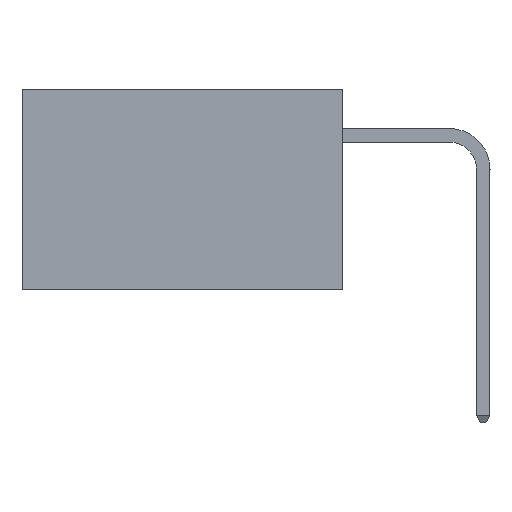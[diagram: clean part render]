
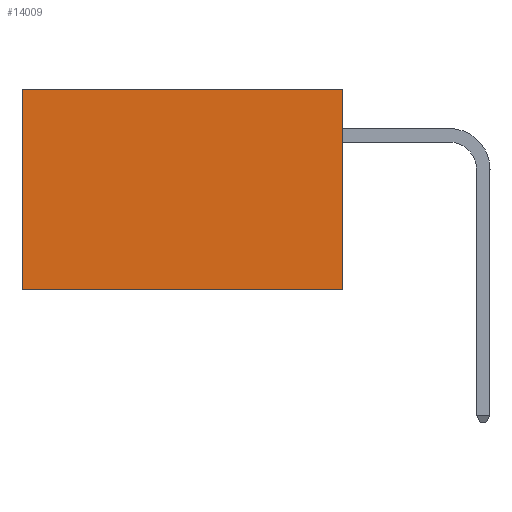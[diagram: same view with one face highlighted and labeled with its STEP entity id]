
A CAD part, left-side view. The second image highlights one B-rep face of the part: STEP entity #14009.
In plain terms, the highlighted planar face has unit normal (-1, 0, 0).
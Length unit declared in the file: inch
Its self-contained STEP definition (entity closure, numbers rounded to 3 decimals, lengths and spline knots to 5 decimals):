
#9 = EDGE_CURVE ( 'NONE', #1036, #16389, #4591, .T. ) ;
#701 = CARTESIAN_POINT ( 'NONE',  ( 0.277, 0., -0.37 ) ) ;
#793 = LINE ( 'NONE', #799, #8828 ) ;
#799 = CARTESIAN_POINT ( 'NONE',  ( 0.277, 0., -0.37 ) ) ;
#1036 = VERTEX_POINT ( 'NONE', #1384 ) ;
#1041 = ORIENTED_EDGE ( 'NONE', *, *, #9, .T. ) ;
#1384 = CARTESIAN_POINT ( 'NONE',  ( 0.277, 0., 0. ) ) ;
#2381 = DIRECTION ( 'NONE',  ( 0., 0., -1. ) ) ;
#2411 = DIRECTION ( 'NONE',  ( 0., 0., -1. ) ) ;
#2448 = DIRECTION ( 'NONE',  ( 0., 1., 0. ) ) ;
#4387 = CARTESIAN_POINT ( 'NONE',  ( 0.277, 0.59, -0.37 ) ) ;
#4591 = LINE ( 'NONE', #5371, #12513 ) ;
#4820 = CARTESIAN_POINT ( 'NONE',  ( 0.277, 0.59, -0.37 ) ) ;
#4919 = VECTOR ( 'NONE', #7154, 39.37008 ) ;
#5371 = CARTESIAN_POINT ( 'NONE',  ( 0.277, 0., 0. ) ) ;
#5419 = LINE ( 'NONE', #14983, #4919 ) ;
#6129 = VERTEX_POINT ( 'NONE', #4387 ) ;
#6445 = EDGE_LOOP ( 'NONE', ( #16163, #11290, #16915, #1041 ) ) ;
#7154 = DIRECTION ( 'NONE',  ( 0., 1., 0. ) ) ;
#8380 = AXIS2_PLACEMENT_3D ( 'NONE', #701, #11923, #2381 ) ;
#8828 = VECTOR ( 'NONE', #2411, 39.37008 ) ;
#9230 = EDGE_CURVE ( 'NONE', #15899, #6129, #5419, .T. ) ;
#10810 = LINE ( 'NONE', #4820, #11299 ) ;
#11290 = ORIENTED_EDGE ( 'NONE', *, *, #9230, .F. ) ;
#11299 = VECTOR ( 'NONE', #17451, 39.37008 ) ;
#11923 = DIRECTION ( 'NONE',  ( 1., 0., 0. ) ) ;
#12513 = VECTOR ( 'NONE', #2448, 39.37008 ) ;
#13425 = PLANE ( 'NONE',  #8380 ) ;
#14009 = ADVANCED_FACE ( 'NONE', ( #19649 ), #13425, .F. ) ;
#14983 = CARTESIAN_POINT ( 'NONE',  ( 0.277, 0., -0.37 ) ) ;
#15899 = VERTEX_POINT ( 'NONE', #20292 ) ;
#16163 = ORIENTED_EDGE ( 'NONE', *, *, #19424, .T. ) ;
#16389 = VERTEX_POINT ( 'NONE', #19787 ) ;
#16915 = ORIENTED_EDGE ( 'NONE', *, *, #19094, .F. ) ;
#17451 = DIRECTION ( 'NONE',  ( 0., 0., -1. ) ) ;
#19094 = EDGE_CURVE ( 'NONE', #1036, #15899, #793, .T. ) ;
#19424 = EDGE_CURVE ( 'NONE', #16389, #6129, #10810, .T. ) ;
#19649 = FACE_OUTER_BOUND ( 'NONE', #6445, .T. ) ;
#19787 = CARTESIAN_POINT ( 'NONE',  ( 0.277, 0.59, 0. ) ) ;
#20292 = CARTESIAN_POINT ( 'NONE',  ( 0.277, 0., -0.37 ) ) ;
